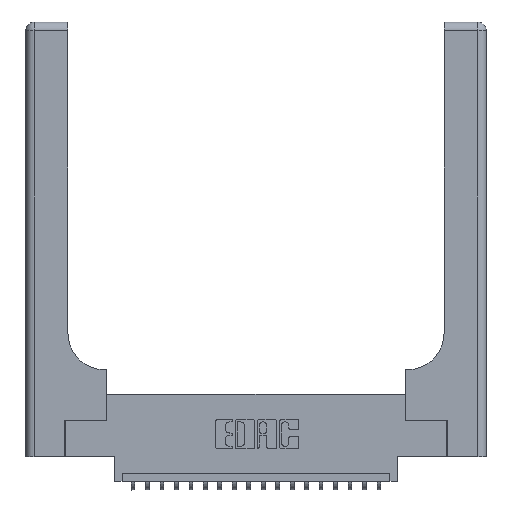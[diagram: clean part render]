
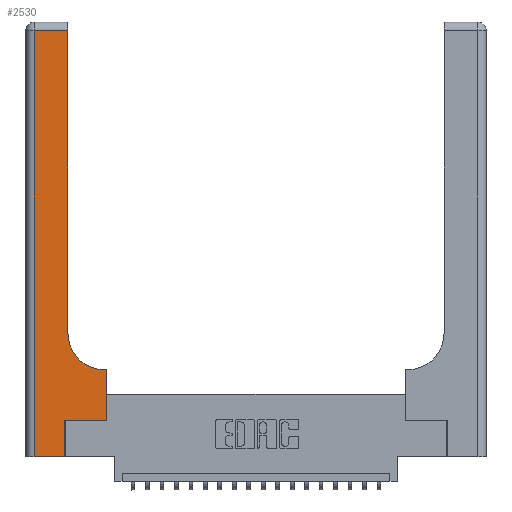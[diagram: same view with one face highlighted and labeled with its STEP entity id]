
A CAD part, top view. The second image highlights one B-rep face of the part: STEP entity #2530.
In plain terms, the highlighted planar face has unit normal (0, 0, 1).
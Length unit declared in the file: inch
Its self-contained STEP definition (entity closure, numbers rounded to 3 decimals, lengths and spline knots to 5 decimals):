
#921 = ORIENTED_EDGE ( 'NONE', *, *, #3750, .T. ) ;
#1064 = CARTESIAN_POINT ( 'NONE',  ( 0.269, 0., 0.37 ) ) ;
#1286 = DIRECTION ( 'NONE',  ( 0., 0., -1. ) ) ;
#1298 = FACE_OUTER_BOUND ( 'NONE', #22167, .T. ) ;
#1510 = EDGE_CURVE ( 'NONE', #17996, #15240, #15538, .T. ) ;
#1886 = CARTESIAN_POINT ( 'NONE',  ( 0.269, 0.25, 0.37 ) ) ;
#1895 = EDGE_CURVE ( 'NONE', #12341, #11640, #15518, .T. ) ;
#2019 = AXIS2_PLACEMENT_3D ( 'NONE', #17135, #10237, #10168 ) ;
#2530 = ADVANCED_FACE ( 'NONE', ( #1298 ), #15056, .F. ) ;
#2673 = DIRECTION ( 'NONE',  ( -1., 0., 0. ) ) ;
#2990 = CARTESIAN_POINT ( 'NONE',  ( 0.06, 2.94, 0.37 ) ) ;
#3399 = EDGE_CURVE ( 'NONE', #18372, #8190, #9024, .T. ) ;
#3466 = VERTEX_POINT ( 'NONE', #4157 ) ;
#3736 = AXIS2_PLACEMENT_3D ( 'NONE', #21715, #1286, #8275 ) ;
#3750 = EDGE_CURVE ( 'NONE', #11640, #3466, #5036, .T. ) ;
#4157 = CARTESIAN_POINT ( 'NONE',  ( 0.2915, 0.85, 0.37 ) ) ;
#5020 = CARTESIAN_POINT ( 'NONE',  ( 0.269, 0.25, 0.37 ) ) ;
#5036 = CIRCLE ( 'NONE', #2019, 0.25 ) ;
#5490 = VERTEX_POINT ( 'NONE', #21898 ) ;
#6272 = EDGE_CURVE ( 'NONE', #8190, #5490, #8867, .T. ) ;
#6338 = CARTESIAN_POINT ( 'NONE',  ( 0., 2.94, 0.37 ) ) ;
#6590 = CARTESIAN_POINT ( 'NONE',  ( 0., 0., 0.37 ) ) ;
#6647 = VECTOR ( 'NONE', #11121, 39.37008 ) ;
#6652 = EDGE_CURVE ( 'NONE', #12509, #17996, #17899, .T. ) ;
#6728 = CARTESIAN_POINT ( 'NONE',  ( 0.2915, 3., 0.37 ) ) ;
#6894 = CARTESIAN_POINT ( 'NONE',  ( 0.5415, 0.6, 0.37 ) ) ;
#7269 = VECTOR ( 'NONE', #12263, 39.37008 ) ;
#7467 = EDGE_CURVE ( 'NONE', #3466, #12509, #18150, .T. ) ;
#7512 = CARTESIAN_POINT ( 'NONE',  ( 0.5585, 0.6, 0.37 ) ) ;
#7659 = ORIENTED_EDGE ( 'NONE', *, *, #7836, .T. ) ;
#7836 = EDGE_CURVE ( 'NONE', #5490, #12341, #9335, .T. ) ;
#7985 = DIRECTION ( 'NONE',  ( -1., 0., 0. ) ) ;
#8190 = VERTEX_POINT ( 'NONE', #5020 ) ;
#8272 = DIRECTION ( 'NONE',  ( 0., -1., 0. ) ) ;
#8275 = DIRECTION ( 'NONE',  ( -1., 0., 0. ) ) ;
#8867 = LINE ( 'NONE', #1886, #7269 ) ;
#9024 = LINE ( 'NONE', #21363, #6647 ) ;
#9335 = LINE ( 'NONE', #12792, #13044 ) ;
#9800 = ORIENTED_EDGE ( 'NONE', *, *, #7467, .T. ) ;
#10168 = DIRECTION ( 'NONE',  ( 1., 0., 0. ) ) ;
#10237 = DIRECTION ( 'NONE',  ( 0., 0., -1. ) ) ;
#10490 = CARTESIAN_POINT ( 'NONE',  ( 0.06, 0., 0.37 ) ) ;
#10786 = ORIENTED_EDGE ( 'NONE', *, *, #6652, .T. ) ;
#10985 = VECTOR ( 'NONE', #7985, 39.37008 ) ;
#11121 = DIRECTION ( 'NONE',  ( 0., 1., 0. ) ) ;
#11280 = CARTESIAN_POINT ( 'NONE',  ( 0.2915, 0.6, 0.37 ) ) ;
#11408 = ORIENTED_EDGE ( 'NONE', *, *, #1510, .T. ) ;
#11640 = VERTEX_POINT ( 'NONE', #6894 ) ;
#12263 = DIRECTION ( 'NONE',  ( 1., 0., 0. ) ) ;
#12341 = VERTEX_POINT ( 'NONE', #7512 ) ;
#12509 = VERTEX_POINT ( 'NONE', #15127 ) ;
#12792 = CARTESIAN_POINT ( 'NONE',  ( 0.5585, 0.25, 0.37 ) ) ;
#12867 = DIRECTION ( 'NONE',  ( 0., 1., 0. ) ) ;
#13044 = VECTOR ( 'NONE', #12867, 39.37008 ) ;
#13641 = DIRECTION ( 'NONE',  ( 0., 1., 0. ) ) ;
#14734 = LINE ( 'NONE', #6590, #16591 ) ;
#14938 = VECTOR ( 'NONE', #13641, 39.37008 ) ;
#15056 = PLANE ( 'NONE',  #3736 ) ;
#15127 = CARTESIAN_POINT ( 'NONE',  ( 0.2915, 2.94, 0.37 ) ) ;
#15240 = VERTEX_POINT ( 'NONE', #10490 ) ;
#15518 = LINE ( 'NONE', #11280, #21668 ) ;
#15538 = LINE ( 'NONE', #22023, #19529 ) ;
#15681 = EDGE_CURVE ( 'NONE', #15240, #18372, #14734, .T. ) ;
#16591 = VECTOR ( 'NONE', #18502, 39.37008 ) ;
#17126 = ORIENTED_EDGE ( 'NONE', *, *, #6272, .T. ) ;
#17135 = CARTESIAN_POINT ( 'NONE',  ( 0.5415, 0.85, 0.37 ) ) ;
#17899 = LINE ( 'NONE', #6338, #10985 ) ;
#17996 = VERTEX_POINT ( 'NONE', #2990 ) ;
#18150 = LINE ( 'NONE', #6728, #14938 ) ;
#18372 = VERTEX_POINT ( 'NONE', #1064 ) ;
#18502 = DIRECTION ( 'NONE',  ( 1., 0., 0. ) ) ;
#19529 = VECTOR ( 'NONE', #8272, 39.37008 ) ;
#20617 = ORIENTED_EDGE ( 'NONE', *, *, #15681, .T. ) ;
#21363 = CARTESIAN_POINT ( 'NONE',  ( 0.269, 0., 0.37 ) ) ;
#21668 = VECTOR ( 'NONE', #2673, 39.37008 ) ;
#21715 = CARTESIAN_POINT ( 'NONE',  ( 0., 3., 0.37 ) ) ;
#21737 = ORIENTED_EDGE ( 'NONE', *, *, #1895, .T. ) ;
#21898 = CARTESIAN_POINT ( 'NONE',  ( 0.5585, 0.25, 0.37 ) ) ;
#21956 = ORIENTED_EDGE ( 'NONE', *, *, #3399, .T. ) ;
#22023 = CARTESIAN_POINT ( 'NONE',  ( 0.06, 3., 0.37 ) ) ;
#22167 = EDGE_LOOP ( 'NONE', ( #9800, #10786, #11408, #20617, #21956, #17126, #7659, #21737, #921 ) ) ;
